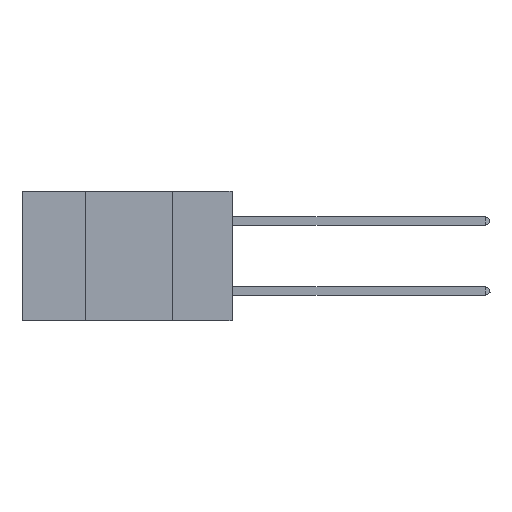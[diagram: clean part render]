
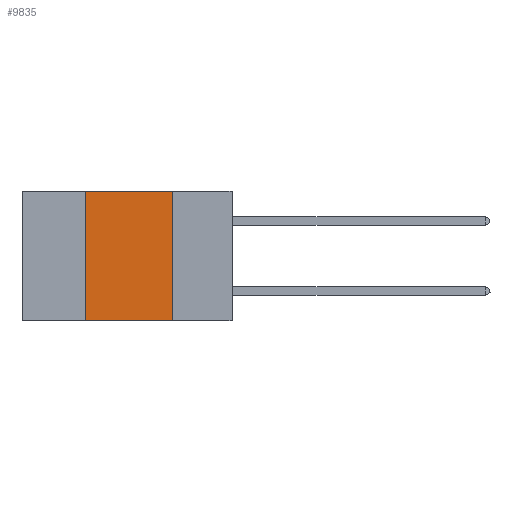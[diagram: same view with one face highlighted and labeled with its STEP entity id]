
A CAD part, left-side view. The second image highlights one B-rep face of the part: STEP entity #9835.
In plain terms, the highlighted planar face has unit normal (-1, 0, 0).
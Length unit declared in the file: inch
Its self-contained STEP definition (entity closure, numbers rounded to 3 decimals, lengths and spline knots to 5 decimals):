
#110 = DIRECTION ( 'NONE',  ( 0., 0., 1. ) ) ;
#143 = CARTESIAN_POINT ( 'NONE',  ( 0., 0.17, -0.37 ) ) ;
#513 = EDGE_CURVE ( 'NONE', #1813, #7868, #12009, .T. ) ;
#761 = CARTESIAN_POINT ( 'NONE',  ( 0., 0.42, 0. ) ) ;
#917 = CARTESIAN_POINT ( 'NONE',  ( 0., 0.6, -0.37 ) ) ;
#998 = VERTEX_POINT ( 'NONE', #761 ) ;
#1170 = EDGE_LOOP ( 'NONE', ( #7790, #3890, #7908, #1273 ) ) ;
#1238 = VECTOR ( 'NONE', #9639, 39.37008 ) ;
#1258 = CARTESIAN_POINT ( 'NONE',  ( 0., 0.42, -0.37 ) ) ;
#1273 = ORIENTED_EDGE ( 'NONE', *, *, #513, .T. ) ;
#1646 = PLANE ( 'NONE',  #4299 ) ;
#1813 = VERTEX_POINT ( 'NONE', #1258 ) ;
#1945 = DIRECTION ( 'NONE',  ( 0., -1., 0. ) ) ;
#3765 = DIRECTION ( 'NONE',  ( 0., 0., -1. ) ) ;
#3858 = EDGE_CURVE ( 'NONE', #9189, #7868, #10716, .T. ) ;
#3890 = ORIENTED_EDGE ( 'NONE', *, *, #9617, .F. ) ;
#4299 = AXIS2_PLACEMENT_3D ( 'NONE', #7685, #9731, #3765 ) ;
#4731 = CARTESIAN_POINT ( 'NONE',  ( 0., 0.17, 0. ) ) ;
#4750 = FACE_OUTER_BOUND ( 'NONE', #1170, .T. ) ;
#5183 = CARTESIAN_POINT ( 'NONE',  ( 0., 0.6, 0. ) ) ;
#5440 = VECTOR ( 'NONE', #110, 39.37008 ) ;
#7526 = EDGE_CURVE ( 'NONE', #1813, #998, #10222, .T. ) ;
#7685 = CARTESIAN_POINT ( 'NONE',  ( 0., 0.6, 0. ) ) ;
#7790 = ORIENTED_EDGE ( 'NONE', *, *, #3858, .F. ) ;
#7868 = VERTEX_POINT ( 'NONE', #143 ) ;
#7908 = ORIENTED_EDGE ( 'NONE', *, *, #7526, .F. ) ;
#8482 = CARTESIAN_POINT ( 'NONE',  ( 0., 0.17, 0. ) ) ;
#9189 = VERTEX_POINT ( 'NONE', #8482 ) ;
#9617 = EDGE_CURVE ( 'NONE', #998, #9189, #12501, .T. ) ;
#9639 = DIRECTION ( 'NONE',  ( 0., 0., -1. ) ) ;
#9731 = DIRECTION ( 'NONE',  ( 1., 0., 0. ) ) ;
#9745 = VECTOR ( 'NONE', #12172, 39.37008 ) ;
#9835 = ADVANCED_FACE ( 'NONE', ( #4750 ), #1646, .F. ) ;
#10222 = LINE ( 'NONE', #12528, #5440 ) ;
#10716 = LINE ( 'NONE', #4731, #1238 ) ;
#12009 = LINE ( 'NONE', #917, #12775 ) ;
#12172 = DIRECTION ( 'NONE',  ( 0., -1., 0. ) ) ;
#12501 = LINE ( 'NONE', #5183, #9745 ) ;
#12528 = CARTESIAN_POINT ( 'NONE',  ( 0., 0.42, 0. ) ) ;
#12775 = VECTOR ( 'NONE', #1945, 39.37008 ) ;
